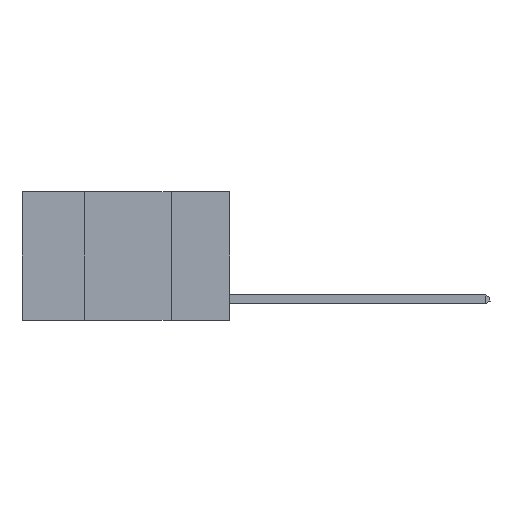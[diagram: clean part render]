
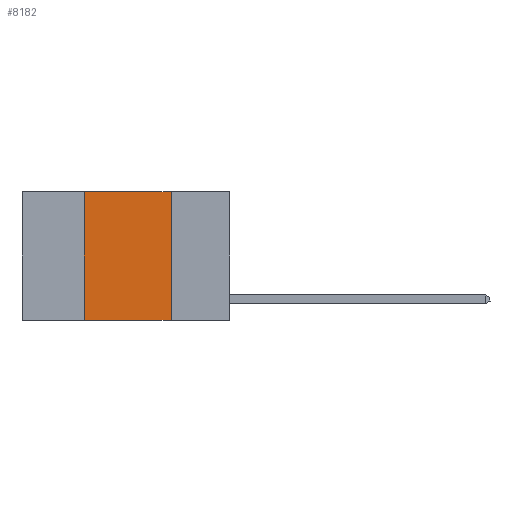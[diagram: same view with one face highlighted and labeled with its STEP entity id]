
A CAD part, left-side view. The second image highlights one B-rep face of the part: STEP entity #8182.
In plain terms, the highlighted planar face has unit normal (-1, 0, 0).
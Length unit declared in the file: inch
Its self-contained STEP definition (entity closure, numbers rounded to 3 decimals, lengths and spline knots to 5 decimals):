
#46 = DIRECTION ( 'NONE',  ( 0., 0., -1. ) ) ;
#211 = CARTESIAN_POINT ( 'NONE',  ( 0., 0.6, 0. ) ) ;
#519 = LINE ( 'NONE', #4594, #5851 ) ;
#643 = EDGE_CURVE ( 'NONE', #6647, #3053, #519, .T. ) ;
#700 = EDGE_CURVE ( 'NONE', #6098, #3053, #951, .T. ) ;
#897 = DIRECTION ( 'NONE',  ( 1., 0., 0. ) ) ;
#951 = LINE ( 'NONE', #5779, #4623 ) ;
#1125 = CARTESIAN_POINT ( 'NONE',  ( 0., 0.17, 0. ) ) ;
#1554 = DIRECTION ( 'NONE',  ( 0., -1., 0. ) ) ;
#1697 = PLANE ( 'NONE',  #5648 ) ;
#2202 = DIRECTION ( 'NONE',  ( 0., -1., 0. ) ) ;
#2334 = CARTESIAN_POINT ( 'NONE',  ( 0., 0.42, 0. ) ) ;
#2351 = DIRECTION ( 'NONE',  ( 0., 0., -1. ) ) ;
#2611 = CARTESIAN_POINT ( 'NONE',  ( 0., 0.17, -0.37 ) ) ;
#2641 = EDGE_CURVE ( 'NONE', #3754, #6098, #7785, .T. ) ;
#3053 = VERTEX_POINT ( 'NONE', #2611 ) ;
#3321 = CARTESIAN_POINT ( 'NONE',  ( 0., 0.42, 0. ) ) ;
#3428 = EDGE_CURVE ( 'NONE', #6647, #3754, #7307, .T. ) ;
#3754 = VERTEX_POINT ( 'NONE', #2334 ) ;
#4087 = VECTOR ( 'NONE', #1554, 39.37008 ) ;
#4337 = ORIENTED_EDGE ( 'NONE', *, *, #2641, .F. ) ;
#4594 = CARTESIAN_POINT ( 'NONE',  ( 0., 0.6, -0.37 ) ) ;
#4623 = VECTOR ( 'NONE', #46, 39.37008 ) ;
#5648 = AXIS2_PLACEMENT_3D ( 'NONE', #211, #897, #2351 ) ;
#5779 = CARTESIAN_POINT ( 'NONE',  ( 0., 0.17, 0. ) ) ;
#5851 = VECTOR ( 'NONE', #2202, 39.37008 ) ;
#6098 = VERTEX_POINT ( 'NONE', #1125 ) ;
#6446 = ORIENTED_EDGE ( 'NONE', *, *, #700, .F. ) ;
#6647 = VERTEX_POINT ( 'NONE', #7652 ) ;
#7307 = LINE ( 'NONE', #3321, #8790 ) ;
#7532 = FACE_OUTER_BOUND ( 'NONE', #7929, .T. ) ;
#7652 = CARTESIAN_POINT ( 'NONE',  ( 0., 0.42, -0.37 ) ) ;
#7672 = DIRECTION ( 'NONE',  ( 0., 0., 1. ) ) ;
#7785 = LINE ( 'NONE', #8606, #4087 ) ;
#7929 = EDGE_LOOP ( 'NONE', ( #6446, #4337, #8063, #9008 ) ) ;
#8063 = ORIENTED_EDGE ( 'NONE', *, *, #3428, .F. ) ;
#8182 = ADVANCED_FACE ( 'NONE', ( #7532 ), #1697, .F. ) ;
#8606 = CARTESIAN_POINT ( 'NONE',  ( 0., 0.6, 0. ) ) ;
#8790 = VECTOR ( 'NONE', #7672, 39.37008 ) ;
#9008 = ORIENTED_EDGE ( 'NONE', *, *, #643, .T. ) ;
